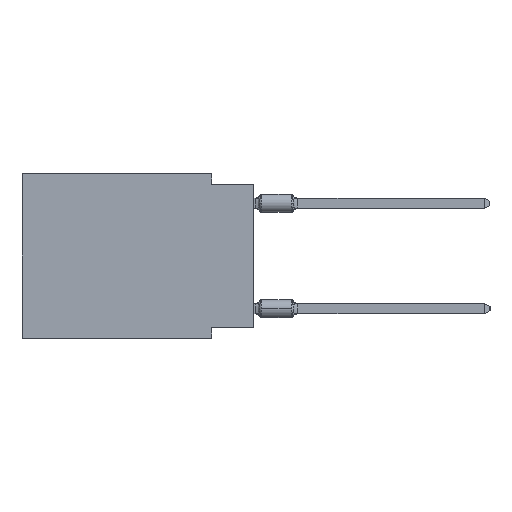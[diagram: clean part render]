
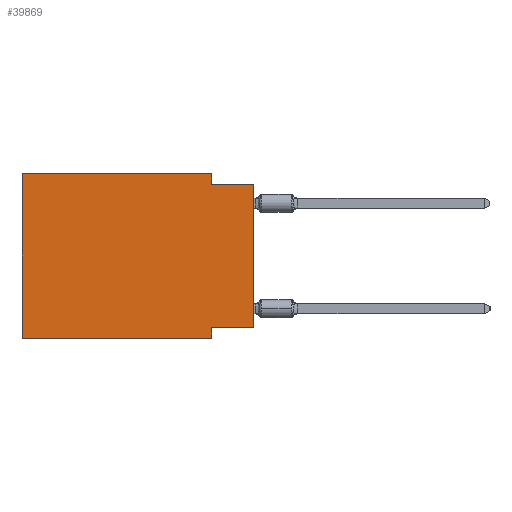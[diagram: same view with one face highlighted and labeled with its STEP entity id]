
A CAD part, left-side view. The second image highlights one B-rep face of the part: STEP entity #39869.
In plain terms, the highlighted planar face has unit normal (-1, 0, 0).
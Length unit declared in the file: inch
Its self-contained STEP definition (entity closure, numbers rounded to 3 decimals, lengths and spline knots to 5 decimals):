
#1311 = LINE ( 'NONE', #3587, #6859 ) ;
#2148 = CARTESIAN_POINT ( 'NONE',  ( 0., 0., -0.365 ) ) ;
#2629 = ORIENTED_EDGE ( 'NONE', *, *, #18511, .F. ) ;
#2927 = AXIS2_PLACEMENT_3D ( 'NONE', #20116, #34111, #24550 ) ;
#3523 = VECTOR ( 'NONE', #7113, 39.37008 ) ;
#3587 = CARTESIAN_POINT ( 'NONE',  ( 0., 0., -0.365 ) ) ;
#4002 = EDGE_CURVE ( 'NONE', #20897, #41266, #20851, .T. ) ;
#4965 = EDGE_CURVE ( 'NONE', #42430, #36579, #34168, .T. ) ;
#5654 = ORIENTED_EDGE ( 'NONE', *, *, #40166, .F. ) ;
#5913 = LINE ( 'NONE', #32760, #41880 ) ;
#6859 = VECTOR ( 'NONE', #38737, 39.37008 ) ;
#7006 = VECTOR ( 'NONE', #25066, 39.37008 ) ;
#7113 = DIRECTION ( 'NONE',  ( 0., 0., -1. ) ) ;
#7548 = CARTESIAN_POINT ( 'NONE',  ( 0., 0.55, -0.39 ) ) ;
#8333 = VECTOR ( 'NONE', #42624, 39.37008 ) ;
#9630 = CARTESIAN_POINT ( 'NONE',  ( 0., 0.1, -0.025 ) ) ;
#10259 = VERTEX_POINT ( 'NONE', #2148 ) ;
#10391 = ORIENTED_EDGE ( 'NONE', *, *, #16389, .F. ) ;
#10401 = CARTESIAN_POINT ( 'NONE',  ( 0., 0.1, -0.365 ) ) ;
#11136 = EDGE_CURVE ( 'NONE', #20897, #41995, #15304, .T. ) ;
#13308 = CARTESIAN_POINT ( 'NONE',  ( 0., 0.1, 0. ) ) ;
#13551 = CARTESIAN_POINT ( 'NONE',  ( 0., 0.55, -0.39 ) ) ;
#14331 = ORIENTED_EDGE ( 'NONE', *, *, #34340, .T. ) ;
#15304 = LINE ( 'NONE', #28843, #16869 ) ;
#15881 = DIRECTION ( 'NONE',  ( 0., -1., 0. ) ) ;
#16389 = EDGE_CURVE ( 'NONE', #32960, #41266, #16969, .T. ) ;
#16869 = VECTOR ( 'NONE', #42140, 39.37008 ) ;
#16969 = LINE ( 'NONE', #36494, #23095 ) ;
#18511 = EDGE_CURVE ( 'NONE', #10259, #32960, #1311, .T. ) ;
#18880 = LINE ( 'NONE', #32435, #8333 ) ;
#19679 = FACE_OUTER_BOUND ( 'NONE', #27250, .T. ) ;
#20116 = CARTESIAN_POINT ( 'NONE',  ( 0., 0.55, 0. ) ) ;
#20851 = LINE ( 'NONE', #7548, #7006 ) ;
#20897 = VERTEX_POINT ( 'NONE', #13551 ) ;
#23095 = VECTOR ( 'NONE', #26970, 39.37008 ) ;
#24016 = DIRECTION ( 'NONE',  ( 0., 0., 1. ) ) ;
#24133 = PLANE ( 'NONE',  #2927 ) ;
#24203 = CARTESIAN_POINT ( 'NONE',  ( 0., 0.1, 0. ) ) ;
#24550 = DIRECTION ( 'NONE',  ( 0., 0., -1. ) ) ;
#24863 = ORIENTED_EDGE ( 'NONE', *, *, #4965, .F. ) ;
#25066 = DIRECTION ( 'NONE',  ( 0., -1., 0. ) ) ;
#26970 = DIRECTION ( 'NONE',  ( 0., 0., -1. ) ) ;
#27250 = EDGE_LOOP ( 'NONE', ( #14331, #5654, #24863, #40472, #30010, #37514, #10391, #2629 ) ) ;
#27332 = CARTESIAN_POINT ( 'NONE',  ( 0., 0., 0. ) ) ;
#27778 = LINE ( 'NONE', #27332, #35886 ) ;
#28843 = CARTESIAN_POINT ( 'NONE',  ( 0., 0.55, 0. ) ) ;
#30010 = ORIENTED_EDGE ( 'NONE', *, *, #11136, .F. ) ;
#31659 = CARTESIAN_POINT ( 'NONE',  ( 0., 0.1, -0.39 ) ) ;
#32435 = CARTESIAN_POINT ( 'NONE',  ( 0., 0.55, 0. ) ) ;
#32760 = CARTESIAN_POINT ( 'NONE',  ( 0., 0., -0.025 ) ) ;
#32960 = VERTEX_POINT ( 'NONE', #10401 ) ;
#34111 = DIRECTION ( 'NONE',  ( 1., 0., 0. ) ) ;
#34168 = LINE ( 'NONE', #13308, #3523 ) ;
#34340 = EDGE_CURVE ( 'NONE', #10259, #38561, #27778, .T. ) ;
#35674 = EDGE_CURVE ( 'NONE', #41995, #42430, #18880, .T. ) ;
#35886 = VECTOR ( 'NONE', #24016, 39.37008 ) ;
#36178 = CARTESIAN_POINT ( 'NONE',  ( 0., 0., -0.025 ) ) ;
#36494 = CARTESIAN_POINT ( 'NONE',  ( 0., 0.1, -0.39 ) ) ;
#36579 = VERTEX_POINT ( 'NONE', #9630 ) ;
#37514 = ORIENTED_EDGE ( 'NONE', *, *, #4002, .T. ) ;
#38561 = VERTEX_POINT ( 'NONE', #36178 ) ;
#38737 = DIRECTION ( 'NONE',  ( 0., 1., 0. ) ) ;
#39869 = ADVANCED_FACE ( 'NONE', ( #19679 ), #24133, .F. ) ;
#40166 = EDGE_CURVE ( 'NONE', #36579, #38561, #5913, .T. ) ;
#40472 = ORIENTED_EDGE ( 'NONE', *, *, #35674, .F. ) ;
#40841 = CARTESIAN_POINT ( 'NONE',  ( 0., 0.55, 0. ) ) ;
#41266 = VERTEX_POINT ( 'NONE', #31659 ) ;
#41880 = VECTOR ( 'NONE', #15881, 39.37008 ) ;
#41995 = VERTEX_POINT ( 'NONE', #40841 ) ;
#42140 = DIRECTION ( 'NONE',  ( 0., 0., 1. ) ) ;
#42430 = VERTEX_POINT ( 'NONE', #24203 ) ;
#42624 = DIRECTION ( 'NONE',  ( 0., -1., 0. ) ) ;
